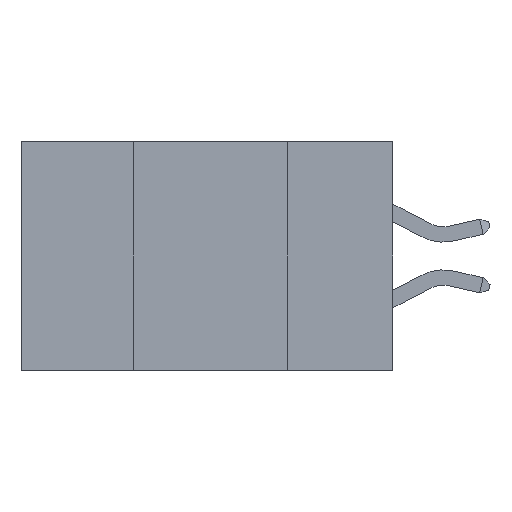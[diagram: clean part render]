
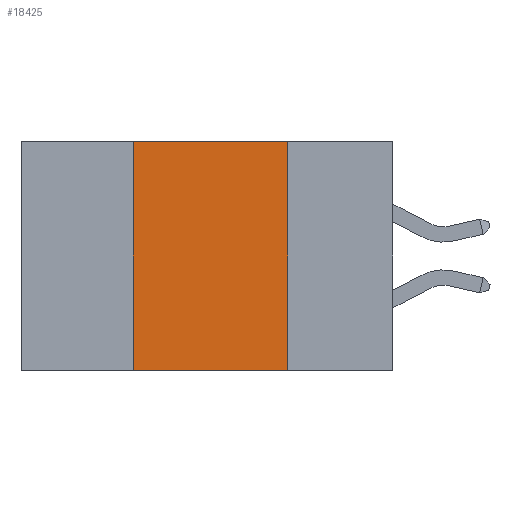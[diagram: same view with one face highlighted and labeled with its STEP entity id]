
A CAD part, left-side view. The second image highlights one B-rep face of the part: STEP entity #18425.
In plain terms, the highlighted planar face has unit normal (-1, 0, 0).
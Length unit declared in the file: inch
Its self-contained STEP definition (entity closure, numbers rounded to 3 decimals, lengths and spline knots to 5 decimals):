
#304 = DIRECTION ( 'NONE',  ( 0., -1., 0. ) ) ;
#1355 = LINE ( 'NONE', #9585, #11291 ) ;
#1490 = ORIENTED_EDGE ( 'NONE', *, *, #13157, .F. ) ;
#1510 = VERTEX_POINT ( 'NONE', #12689 ) ;
#1517 = PLANE ( 'NONE',  #7599 ) ;
#2031 = EDGE_CURVE ( 'NONE', #1510, #18437, #20172, .T. ) ;
#3221 = EDGE_CURVE ( 'NONE', #7820, #17278, #21560, .T. ) ;
#3420 = DIRECTION ( 'NONE',  ( 1., 0., 0. ) ) ;
#3979 = DIRECTION ( 'NONE',  ( 0., 0., -1. ) ) ;
#4363 = EDGE_LOOP ( 'NONE', ( #4827, #21456, #1490, #9896 ) ) ;
#4827 = ORIENTED_EDGE ( 'NONE', *, *, #14376, .F. ) ;
#6106 = CARTESIAN_POINT ( 'NONE',  ( 0., 0.42, 0. ) ) ;
#6581 = DIRECTION ( 'NONE',  ( 0., -1., 0. ) ) ;
#7599 = AXIS2_PLACEMENT_3D ( 'NONE', #14487, #3420, #16314 ) ;
#7820 = VERTEX_POINT ( 'NONE', #19515 ) ;
#8009 = DIRECTION ( 'NONE',  ( 0., 0., 1. ) ) ;
#9585 = CARTESIAN_POINT ( 'NONE',  ( 0., 0.17, 0. ) ) ;
#9832 = VECTOR ( 'NONE', #304, 39.37008 ) ;
#9896 = ORIENTED_EDGE ( 'NONE', *, *, #3221, .T. ) ;
#11183 = CARTESIAN_POINT ( 'NONE',  ( 0., 0.6, 0. ) ) ;
#11291 = VECTOR ( 'NONE', #3979, 39.37008 ) ;
#12689 = CARTESIAN_POINT ( 'NONE',  ( 0., 0.42, 0. ) ) ;
#13157 = EDGE_CURVE ( 'NONE', #7820, #1510, #18828, .T. ) ;
#14376 = EDGE_CURVE ( 'NONE', #18437, #17278, #1355, .T. ) ;
#14487 = CARTESIAN_POINT ( 'NONE',  ( 0., 0.6, 0. ) ) ;
#15107 = FACE_OUTER_BOUND ( 'NONE', #4363, .T. ) ;
#16234 = CARTESIAN_POINT ( 'NONE',  ( 0., 0.17, 0. ) ) ;
#16314 = DIRECTION ( 'NONE',  ( 0., 0., -1. ) ) ;
#16632 = VECTOR ( 'NONE', #6581, 39.37008 ) ;
#17278 = VERTEX_POINT ( 'NONE', #23944 ) ;
#18425 = ADVANCED_FACE ( 'NONE', ( #15107 ), #1517, .F. ) ;
#18437 = VERTEX_POINT ( 'NONE', #16234 ) ;
#18828 = LINE ( 'NONE', #6106, #19407 ) ;
#19407 = VECTOR ( 'NONE', #8009, 39.37008 ) ;
#19515 = CARTESIAN_POINT ( 'NONE',  ( 0., 0.42, -0.37 ) ) ;
#20172 = LINE ( 'NONE', #11183, #9832 ) ;
#21242 = CARTESIAN_POINT ( 'NONE',  ( 0., 0.6, -0.37 ) ) ;
#21456 = ORIENTED_EDGE ( 'NONE', *, *, #2031, .F. ) ;
#21560 = LINE ( 'NONE', #21242, #16632 ) ;
#23944 = CARTESIAN_POINT ( 'NONE',  ( 0., 0.17, -0.37 ) ) ;
